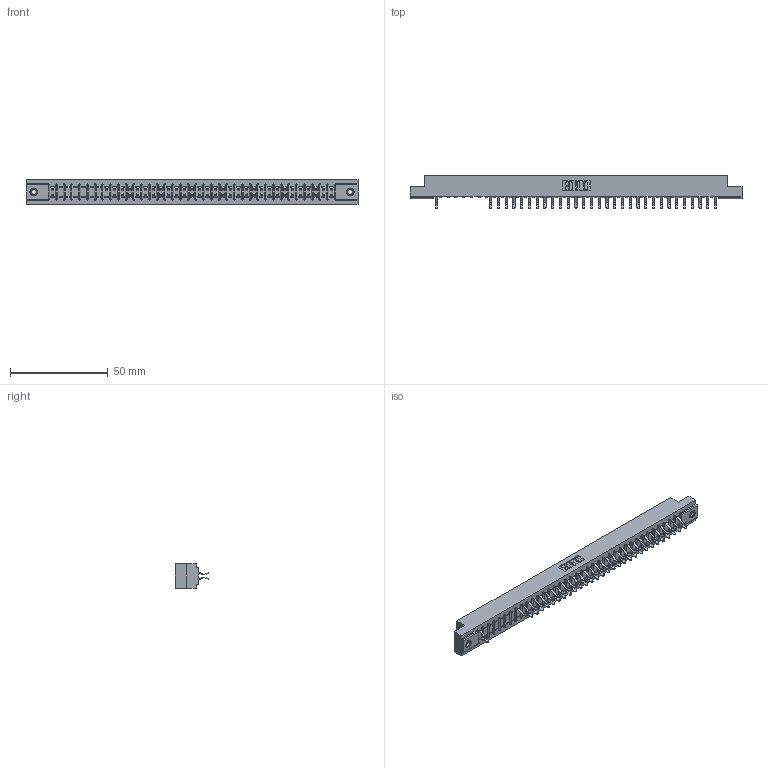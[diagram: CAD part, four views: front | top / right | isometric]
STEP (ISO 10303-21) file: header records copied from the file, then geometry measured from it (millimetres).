
FILE_DESCRIPTION (( 'STEP AP203' ), '1' );
FILE_NAME ('307-074-556-207.STEP', '2018-08-06T16:23:59', ( '' ), ( '' ), 'SwSTEP 2.0', 'SolidWorks 2016', '' );
FILE_SCHEMA (( 'CONFIG_CONTROL_DESIGN' ));
Length unit declared in the file: inch
Products named in the file (4): 307 Part_.156 Dia Mounting Holes; 307-290-001_556; 345-250-001_345-250-005-103; 307-074-556-207
Assembly tree (64 placements, depth 2):
  307-074-556-207
    307 Part_.156 Dia Mounting Holes
    307-290-001_556  x61
    345-250-001_345-250-005-103  x2
Bounding box: 169.62 x 16.97 x 12.7 mm (x, y, z)
Volume: 17808.9 mm3; surface area: 20456.6 mm2
Topology: 64 solids, 64 shells, 3396 faces, 9537 edges, 6166 vertices
Faces by surface type: plane 2193, cylinder 1111, sphere 76, cone 12, torus 4
Entity records: 34393 total; most frequent: CARTESIAN_POINT 5667, ORIENTED_EDGE 5622, DIRECTION 5549, EDGE_CURVE 2811, VECTOR 2153, LINE 2153, VERTEX_POINT 1816, AXIS2_PLACEMENT_3D 1698
